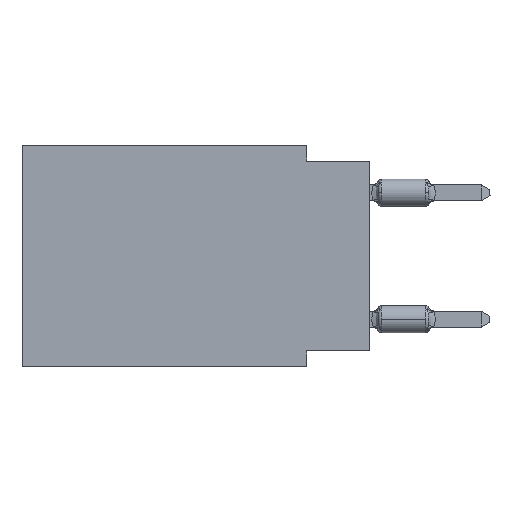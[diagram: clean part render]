
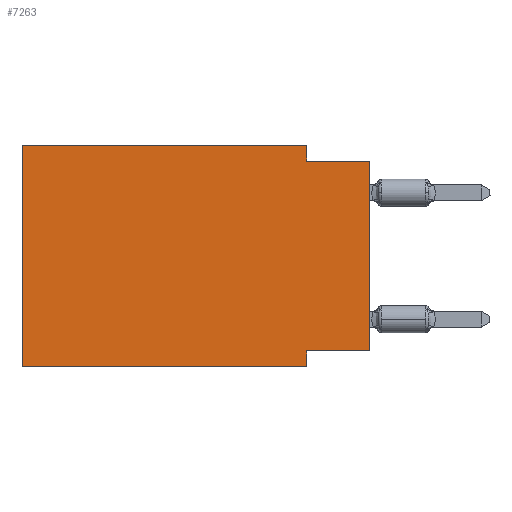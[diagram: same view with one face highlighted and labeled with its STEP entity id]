
A CAD part, left-side view. The second image highlights one B-rep face of the part: STEP entity #7263.
In plain terms, the highlighted planar face has unit normal (-1, 0, 0).
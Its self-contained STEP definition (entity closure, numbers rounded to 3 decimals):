
#60 = DIRECTION ( 'NONE',  ( 0., -1., 0. ) ) ;
#501 = FACE_OUTER_BOUND ( 'NONE', #3651, .T. ) ;
#1040 = LINE ( 'NONE', #4971, #9371 ) ;
#1071 = LINE ( 'NONE', #8845, #13013 ) ;
#1133 = DIRECTION ( 'NONE',  ( 0., 1., 0. ) ) ;
#1676 = CARTESIAN_POINT ( 'NONE',  ( 0., 0., -0.635 ) ) ;
#1957 = CARTESIAN_POINT ( 'NONE',  ( 0., 0., 0. ) ) ;
#2736 = PLANE ( 'NONE',  #9423 ) ;
#3364 = DIRECTION ( 'NONE',  ( 0., -1., 0. ) ) ;
#3486 = CARTESIAN_POINT ( 'NONE',  ( 0., 2.54, -8.89 ) ) ;
#3651 = EDGE_LOOP ( 'NONE', ( #7055, #14988, #6080, #8950, #8957, #12929, #15206, #6470 ) ) ;
#3820 = CARTESIAN_POINT ( 'NONE',  ( 0., 13.97, 0. ) ) ;
#3934 = EDGE_CURVE ( 'NONE', #16332, #9019, #15670, .T. ) ;
#4112 = EDGE_CURVE ( 'NONE', #16332, #10959, #4203, .T. ) ;
#4203 = LINE ( 'NONE', #9513, #11158 ) ;
#4255 = DIRECTION ( 'NONE',  ( 0., 0., -1. ) ) ;
#4653 = LINE ( 'NONE', #10041, #14000 ) ;
#4889 = EDGE_CURVE ( 'NONE', #15111, #14217, #6665, .T. ) ;
#4971 = CARTESIAN_POINT ( 'NONE',  ( 0., 0., -8.255 ) ) ;
#6080 = ORIENTED_EDGE ( 'NONE', *, *, #4889, .F. ) ;
#6468 = DIRECTION ( 'NONE',  ( 0., 0., -1. ) ) ;
#6470 = ORIENTED_EDGE ( 'NONE', *, *, #11736, .F. ) ;
#6592 = DIRECTION ( 'NONE',  ( 0., 0., -1. ) ) ;
#6665 = LINE ( 'NONE', #9471, #7889 ) ;
#6726 = EDGE_CURVE ( 'NONE', #13052, #9019, #1071, .T. ) ;
#7055 = ORIENTED_EDGE ( 'NONE', *, *, #7880, .T. ) ;
#7263 = ADVANCED_FACE ( 'NONE', ( #501 ), #2736, .F. ) ;
#7639 = VERTEX_POINT ( 'NONE', #8496 ) ;
#7814 = CARTESIAN_POINT ( 'NONE',  ( 0., 13.97, -8.89 ) ) ;
#7880 = EDGE_CURVE ( 'NONE', #7639, #11005, #11289, .T. ) ;
#7889 = VECTOR ( 'NONE', #6592, 1000. ) ;
#8496 = CARTESIAN_POINT ( 'NONE',  ( 0., 0., -8.255 ) ) ;
#8845 = CARTESIAN_POINT ( 'NONE',  ( 0., 2.54, -8.89 ) ) ;
#8950 = ORIENTED_EDGE ( 'NONE', *, *, #11159, .F. ) ;
#8957 = ORIENTED_EDGE ( 'NONE', *, *, #4112, .F. ) ;
#9019 = VERTEX_POINT ( 'NONE', #3486 ) ;
#9371 = VECTOR ( 'NONE', #1133, 1000. ) ;
#9422 = DIRECTION ( 'NONE',  ( 0., 0., 1. ) ) ;
#9423 = AXIS2_PLACEMENT_3D ( 'NONE', #10773, #16046, #4255 ) ;
#9471 = CARTESIAN_POINT ( 'NONE',  ( 0., 2.54, 0. ) ) ;
#9513 = CARTESIAN_POINT ( 'NONE',  ( 0., 13.97, 0. ) ) ;
#9649 = EDGE_CURVE ( 'NONE', #14217, #11005, #11771, .T. ) ;
#10041 = CARTESIAN_POINT ( 'NONE',  ( 0., 13.97, 0. ) ) ;
#10773 = CARTESIAN_POINT ( 'NONE',  ( 0., 13.97, 0. ) ) ;
#10781 = CARTESIAN_POINT ( 'NONE',  ( 0., 13.97, -8.89 ) ) ;
#10959 = VERTEX_POINT ( 'NONE', #3820 ) ;
#11005 = VERTEX_POINT ( 'NONE', #1676 ) ;
#11158 = VECTOR ( 'NONE', #9422, 1000. ) ;
#11159 = EDGE_CURVE ( 'NONE', #10959, #15111, #4653, .T. ) ;
#11289 = LINE ( 'NONE', #1957, #11900 ) ;
#11736 = EDGE_CURVE ( 'NONE', #7639, #13052, #1040, .T. ) ;
#11771 = LINE ( 'NONE', #15683, #15484 ) ;
#11900 = VECTOR ( 'NONE', #12390, 1000. ) ;
#11930 = CARTESIAN_POINT ( 'NONE',  ( 0., 2.54, -0.635 ) ) ;
#12390 = DIRECTION ( 'NONE',  ( 0., 0., 1. ) ) ;
#12761 = VECTOR ( 'NONE', #14046, 1000. ) ;
#12929 = ORIENTED_EDGE ( 'NONE', *, *, #3934, .T. ) ;
#13013 = VECTOR ( 'NONE', #6468, 1000. ) ;
#13042 = CARTESIAN_POINT ( 'NONE',  ( 0., 2.54, -8.255 ) ) ;
#13052 = VERTEX_POINT ( 'NONE', #13042 ) ;
#14000 = VECTOR ( 'NONE', #3364, 1000. ) ;
#14046 = DIRECTION ( 'NONE',  ( 0., -1., 0. ) ) ;
#14217 = VERTEX_POINT ( 'NONE', #11930 ) ;
#14672 = CARTESIAN_POINT ( 'NONE',  ( 0., 2.54, 0. ) ) ;
#14988 = ORIENTED_EDGE ( 'NONE', *, *, #9649, .F. ) ;
#15111 = VERTEX_POINT ( 'NONE', #14672 ) ;
#15206 = ORIENTED_EDGE ( 'NONE', *, *, #6726, .F. ) ;
#15484 = VECTOR ( 'NONE', #60, 1000. ) ;
#15670 = LINE ( 'NONE', #7814, #12761 ) ;
#15683 = CARTESIAN_POINT ( 'NONE',  ( 0., 0., -0.635 ) ) ;
#16046 = DIRECTION ( 'NONE',  ( 1., 0., 0. ) ) ;
#16332 = VERTEX_POINT ( 'NONE', #10781 ) ;
